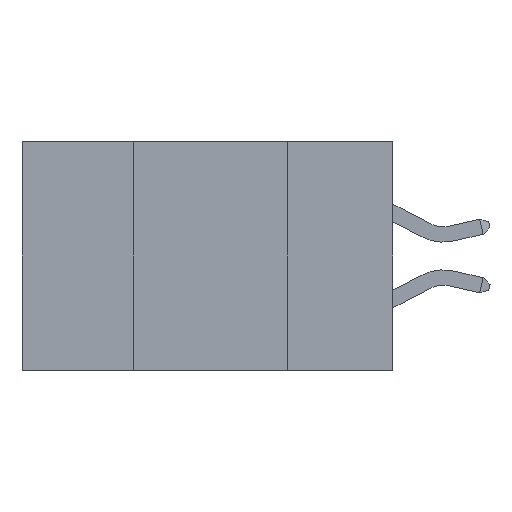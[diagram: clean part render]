
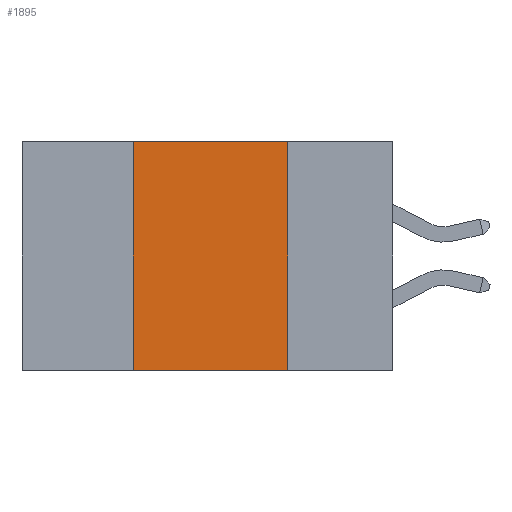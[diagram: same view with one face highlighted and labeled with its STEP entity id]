
A CAD part, left-side view. The second image highlights one B-rep face of the part: STEP entity #1895.
In plain terms, the highlighted planar face has unit normal (-1, 0, 0).
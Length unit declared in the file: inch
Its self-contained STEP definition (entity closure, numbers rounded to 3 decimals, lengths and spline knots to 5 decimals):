
#179 = FACE_OUTER_BOUND ( 'NONE', #7125, .T. ) ;
#552 = CARTESIAN_POINT ( 'NONE',  ( 0., 0.6, -0.37 ) ) ;
#927 = VERTEX_POINT ( 'NONE', #4700 ) ;
#1314 = VERTEX_POINT ( 'NONE', #12848 ) ;
#1860 = EDGE_CURVE ( 'NONE', #927, #19722, #19842, .T. ) ;
#1895 = ADVANCED_FACE ( 'NONE', ( #179 ), #16547, .F. ) ;
#2325 = ORIENTED_EDGE ( 'NONE', *, *, #12822, .F. ) ;
#2815 = ORIENTED_EDGE ( 'NONE', *, *, #20192, .T. ) ;
#4700 = CARTESIAN_POINT ( 'NONE',  ( 0., 0.42, 0. ) ) ;
#5563 = VECTOR ( 'NONE', #12041, 39.37008 ) ;
#5592 = AXIS2_PLACEMENT_3D ( 'NONE', #5642, #13329, #8844 ) ;
#5642 = CARTESIAN_POINT ( 'NONE',  ( 0., 0.6, 0. ) ) ;
#7125 = EDGE_LOOP ( 'NONE', ( #2325, #19172, #19595, #2815 ) ) ;
#7356 = DIRECTION ( 'NONE',  ( 0., 0., -1. ) ) ;
#8086 = LINE ( 'NONE', #552, #13491 ) ;
#8251 = LINE ( 'NONE', #10641, #9980 ) ;
#8844 = DIRECTION ( 'NONE',  ( 0., 0., -1. ) ) ;
#9980 = VECTOR ( 'NONE', #7356, 39.37008 ) ;
#10641 = CARTESIAN_POINT ( 'NONE',  ( 0., 0.17, 0. ) ) ;
#11466 = DIRECTION ( 'NONE',  ( 0., -1., 0. ) ) ;
#11884 = EDGE_CURVE ( 'NONE', #1314, #927, #13920, .T. ) ;
#12041 = DIRECTION ( 'NONE',  ( 0., 0., 1. ) ) ;
#12573 = VERTEX_POINT ( 'NONE', #20275 ) ;
#12822 = EDGE_CURVE ( 'NONE', #19722, #12573, #8251, .T. ) ;
#12848 = CARTESIAN_POINT ( 'NONE',  ( 0., 0.42, -0.37 ) ) ;
#13329 = DIRECTION ( 'NONE',  ( 1., 0., 0. ) ) ;
#13431 = CARTESIAN_POINT ( 'NONE',  ( 0., 0.42, 0. ) ) ;
#13491 = VECTOR ( 'NONE', #14494, 39.37008 ) ;
#13920 = LINE ( 'NONE', #13431, #5563 ) ;
#14494 = DIRECTION ( 'NONE',  ( 0., -1., 0. ) ) ;
#15183 = VECTOR ( 'NONE', #11466, 39.37008 ) ;
#16128 = CARTESIAN_POINT ( 'NONE',  ( 0., 0.6, 0. ) ) ;
#16547 = PLANE ( 'NONE',  #5592 ) ;
#19172 = ORIENTED_EDGE ( 'NONE', *, *, #1860, .F. ) ;
#19201 = CARTESIAN_POINT ( 'NONE',  ( 0., 0.17, 0. ) ) ;
#19595 = ORIENTED_EDGE ( 'NONE', *, *, #11884, .F. ) ;
#19722 = VERTEX_POINT ( 'NONE', #19201 ) ;
#19842 = LINE ( 'NONE', #16128, #15183 ) ;
#20192 = EDGE_CURVE ( 'NONE', #1314, #12573, #8086, .T. ) ;
#20275 = CARTESIAN_POINT ( 'NONE',  ( 0., 0.17, -0.37 ) ) ;
